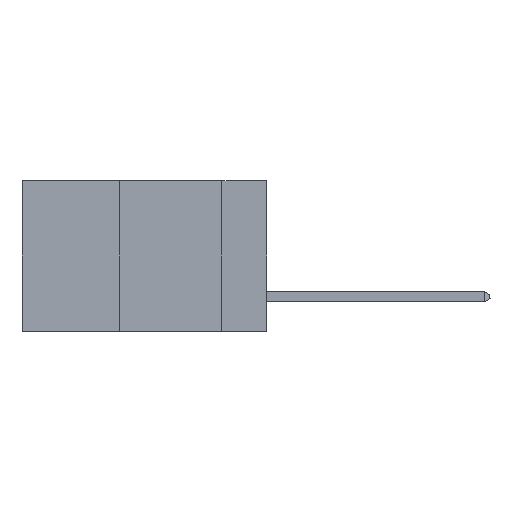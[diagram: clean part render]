
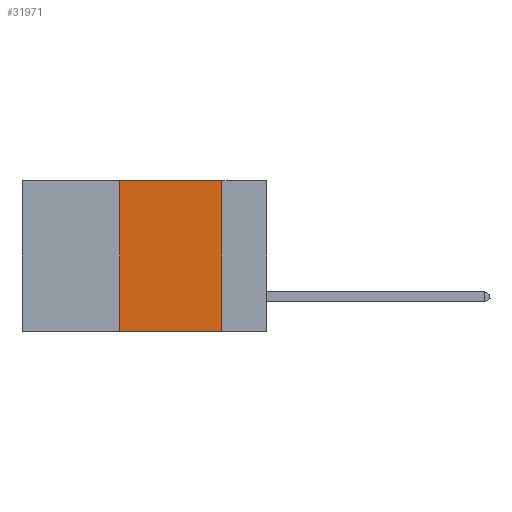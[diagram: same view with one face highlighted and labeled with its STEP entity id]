
A CAD part, left-side view. The second image highlights one B-rep face of the part: STEP entity #31971.
In plain terms, the highlighted planar face has unit normal (-1, 0, 0).
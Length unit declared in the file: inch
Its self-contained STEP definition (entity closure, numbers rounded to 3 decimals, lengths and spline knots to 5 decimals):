
#1113 = CARTESIAN_POINT ( 'NONE',  ( 0., 0.36, 0. ) ) ;
#1405 = LINE ( 'NONE', #1113, #44816 ) ;
#2526 = CARTESIAN_POINT ( 'NONE',  ( 0., 0.6, 0. ) ) ;
#4117 = ORIENTED_EDGE ( 'NONE', *, *, #26541, .F. ) ;
#4604 = LINE ( 'NONE', #11684, #34165 ) ;
#6068 = CARTESIAN_POINT ( 'NONE',  ( 0., 0.6, 0. ) ) ;
#7215 = DIRECTION ( 'NONE',  ( 0., -1., 0. ) ) ;
#8280 = ORIENTED_EDGE ( 'NONE', *, *, #32051, .T. ) ;
#8878 = ORIENTED_EDGE ( 'NONE', *, *, #35601, .F. ) ;
#8897 = DIRECTION ( 'NONE',  ( 0., 0., 1. ) ) ;
#9429 = DIRECTION ( 'NONE',  ( 0., 0., -1. ) ) ;
#9891 = VERTEX_POINT ( 'NONE', #29846 ) ;
#11684 = CARTESIAN_POINT ( 'NONE',  ( 0., 0.6, -0.37 ) ) ;
#13094 = VECTOR ( 'NONE', #33263, 39.37008 ) ;
#15450 = CARTESIAN_POINT ( 'NONE',  ( 0., 0.36, -0.37 ) ) ;
#15592 = LINE ( 'NONE', #2526, #13094 ) ;
#19784 = ORIENTED_EDGE ( 'NONE', *, *, #19959, .F. ) ;
#19959 = EDGE_CURVE ( 'NONE', #43706, #9891, #37810, .T. ) ;
#24631 = DIRECTION ( 'NONE',  ( 1., 0., 0. ) ) ;
#25169 = PLANE ( 'NONE',  #37966 ) ;
#26541 = EDGE_CURVE ( 'NONE', #45143, #49576, #1405, .T. ) ;
#27446 = FACE_OUTER_BOUND ( 'NONE', #38709, .T. ) ;
#29846 = CARTESIAN_POINT ( 'NONE',  ( 0., 0.11, -0.37 ) ) ;
#31971 = ADVANCED_FACE ( 'NONE', ( #27446 ), #25169, .F. ) ;
#32051 = EDGE_CURVE ( 'NONE', #45143, #9891, #4604, .T. ) ;
#33175 = CARTESIAN_POINT ( 'NONE',  ( 0., 0.11, 0. ) ) ;
#33263 = DIRECTION ( 'NONE',  ( 0., -1., 0. ) ) ;
#33548 = CARTESIAN_POINT ( 'NONE',  ( 0., 0.11, 0. ) ) ;
#34165 = VECTOR ( 'NONE', #7215, 39.37008 ) ;
#35601 = EDGE_CURVE ( 'NONE', #49576, #43706, #15592, .T. ) ;
#36076 = DIRECTION ( 'NONE',  ( 0., 0., -1. ) ) ;
#37810 = LINE ( 'NONE', #33175, #46206 ) ;
#37966 = AXIS2_PLACEMENT_3D ( 'NONE', #6068, #24631, #36076 ) ;
#38709 = EDGE_LOOP ( 'NONE', ( #19784, #8878, #4117, #8280 ) ) ;
#42891 = CARTESIAN_POINT ( 'NONE',  ( 0., 0.36, 0. ) ) ;
#43706 = VERTEX_POINT ( 'NONE', #33548 ) ;
#44816 = VECTOR ( 'NONE', #8897, 39.37008 ) ;
#45143 = VERTEX_POINT ( 'NONE', #15450 ) ;
#46206 = VECTOR ( 'NONE', #9429, 39.37008 ) ;
#49576 = VERTEX_POINT ( 'NONE', #42891 ) ;
